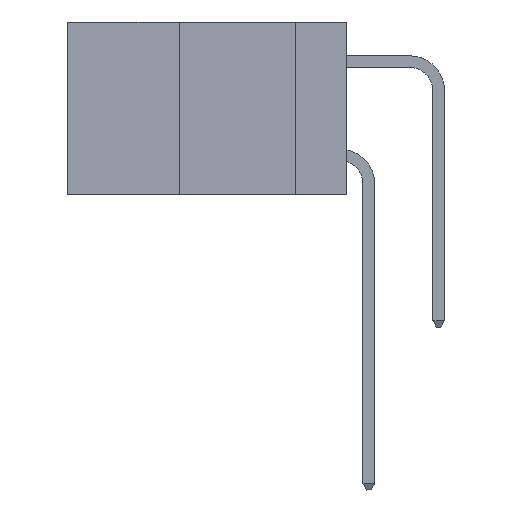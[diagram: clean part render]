
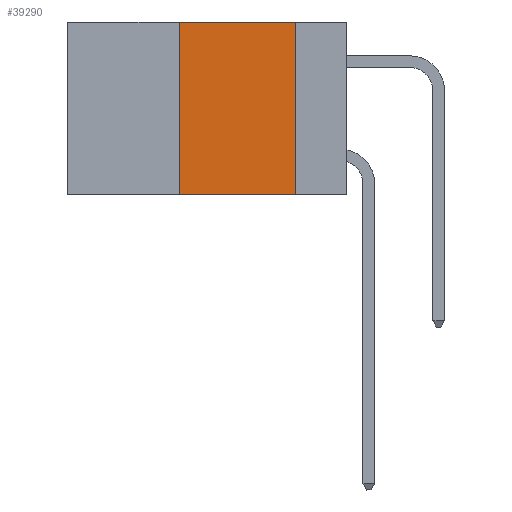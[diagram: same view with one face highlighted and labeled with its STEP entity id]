
A CAD part, left-side view. The second image highlights one B-rep face of the part: STEP entity #39290.
In plain terms, the highlighted planar face has unit normal (-1, 0, 0).
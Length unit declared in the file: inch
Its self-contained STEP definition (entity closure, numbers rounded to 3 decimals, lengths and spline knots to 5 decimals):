
#231 = FACE_OUTER_BOUND ( 'NONE', #4352, .T. ) ;
#2918 = DIRECTION ( 'NONE',  ( 0., 0., 1. ) ) ;
#4352 = EDGE_LOOP ( 'NONE', ( #10804, #32392, #40294, #24954 ) ) ;
#5163 = CARTESIAN_POINT ( 'NONE',  ( 0., 0.36, 0. ) ) ;
#9033 = EDGE_CURVE ( 'NONE', #28963, #19329, #21732, .T. ) ;
#9439 = DIRECTION ( 'NONE',  ( 0., -1., 0. ) ) ;
#10804 = ORIENTED_EDGE ( 'NONE', *, *, #29920, .F. ) ;
#15968 = CARTESIAN_POINT ( 'NONE',  ( 0., 0.6, -0.37 ) ) ;
#16249 = PLANE ( 'NONE',  #42695 ) ;
#17046 = DIRECTION ( 'NONE',  ( 0., -1., 0. ) ) ;
#17445 = EDGE_CURVE ( 'NONE', #32678, #40946, #36281, .T. ) ;
#19329 = VERTEX_POINT ( 'NONE', #38736 ) ;
#19538 = CARTESIAN_POINT ( 'NONE',  ( 0., 0.36, -0.37 ) ) ;
#21732 = LINE ( 'NONE', #15968, #37873 ) ;
#24671 = EDGE_CURVE ( 'NONE', #28963, #32678, #35582, .T. ) ;
#24954 = ORIENTED_EDGE ( 'NONE', *, *, #9033, .T. ) ;
#25858 = CARTESIAN_POINT ( 'NONE',  ( 0., 0.36, 0. ) ) ;
#26267 = DIRECTION ( 'NONE',  ( 0., 0., -1. ) ) ;
#27199 = CARTESIAN_POINT ( 'NONE',  ( 0., 0.6, 0. ) ) ;
#27872 = CARTESIAN_POINT ( 'NONE',  ( 0., 0.11, 0. ) ) ;
#28963 = VERTEX_POINT ( 'NONE', #19538 ) ;
#29920 = EDGE_CURVE ( 'NONE', #40946, #19329, #37738, .T. ) ;
#31382 = VECTOR ( 'NONE', #2918, 39.37008 ) ;
#32392 = ORIENTED_EDGE ( 'NONE', *, *, #17445, .F. ) ;
#32678 = VERTEX_POINT ( 'NONE', #5163 ) ;
#33410 = CARTESIAN_POINT ( 'NONE',  ( 0., 0.6, 0. ) ) ;
#35582 = LINE ( 'NONE', #25858, #31382 ) ;
#36281 = LINE ( 'NONE', #27199, #40475 ) ;
#36701 = VECTOR ( 'NONE', #37650, 39.37008 ) ;
#37650 = DIRECTION ( 'NONE',  ( 0., 0., -1. ) ) ;
#37738 = LINE ( 'NONE', #27872, #36701 ) ;
#37873 = VECTOR ( 'NONE', #9439, 39.37008 ) ;
#38736 = CARTESIAN_POINT ( 'NONE',  ( 0., 0.11, -0.37 ) ) ;
#39290 = ADVANCED_FACE ( 'NONE', ( #231 ), #16249, .F. ) ;
#40294 = ORIENTED_EDGE ( 'NONE', *, *, #24671, .F. ) ;
#40475 = VECTOR ( 'NONE', #17046, 39.37008 ) ;
#40946 = VERTEX_POINT ( 'NONE', #41753 ) ;
#41753 = CARTESIAN_POINT ( 'NONE',  ( 0., 0.11, 0. ) ) ;
#42695 = AXIS2_PLACEMENT_3D ( 'NONE', #33410, #43075, #26267 ) ;
#43075 = DIRECTION ( 'NONE',  ( 1., 0., 0. ) ) ;
